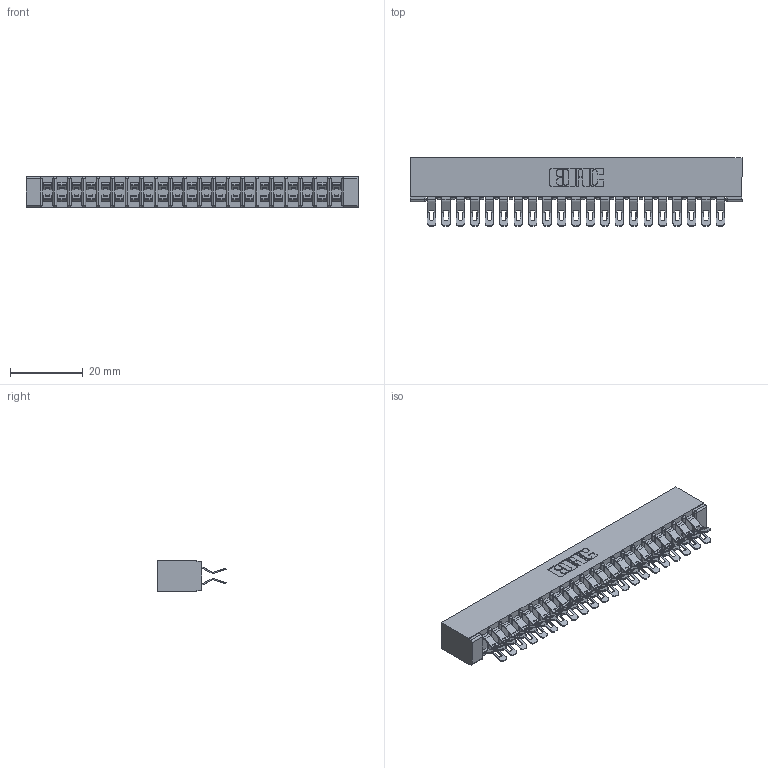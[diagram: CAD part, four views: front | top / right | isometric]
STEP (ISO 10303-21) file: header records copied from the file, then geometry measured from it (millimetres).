
FILE_DESCRIPTION (( 'STEP AP203' ), '1' );
FILE_NAME ('307-042-555-201.STEP', '2019-09-06T06:43:48', ( '' ), ( '' ), 'SwSTEP 2.0', 'SolidWorks 2016', '' );
FILE_SCHEMA (( 'CONFIG_CONTROL_DESIGN' ));
Length unit declared in the file: inch
Products named in the file (3): 307-290-001_555; 307 Part_No Mounting Lugs; 307-042-555-201
Assembly tree (43 placements, depth 2):
  307-042-555-201
    307 Part_No Mounting Lugs
    307-290-001_555  x42
Bounding box: 91.08 x 18.75 x 8.71 mm (x, y, z)
Volume: 6316.3 mm3; surface area: 12265.7 mm2
Topology: 43 solids, 43 shells, 2694 faces, 7901 edges, 5150 vertices
Faces by surface type: plane 1494, cylinder 1156, sphere 44
Entity records: 21523 total; most frequent: CARTESIAN_POINT 3529, ORIENTED_EDGE 3496, DIRECTION 3472, EDGE_CURVE 1748, VECTOR 1322, LINE 1322, VERTEX_POINT 1132, AXIS2_PLACEMENT_3D 1075
